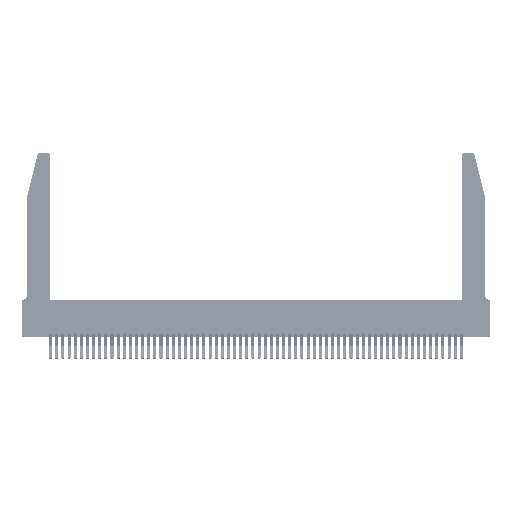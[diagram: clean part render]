
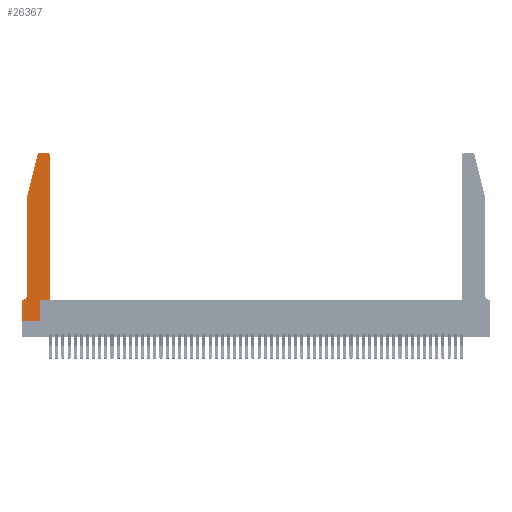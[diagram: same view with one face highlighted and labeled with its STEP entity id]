
A CAD part, top view. The second image highlights one B-rep face of the part: STEP entity #26367.
In plain terms, the highlighted planar face has unit normal (0, 0, 1).
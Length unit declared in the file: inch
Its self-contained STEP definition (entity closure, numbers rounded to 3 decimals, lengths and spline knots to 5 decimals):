
#1747 = ORIENTED_EDGE ( 'NONE', *, *, #37075, .T. ) ;
#2372 = VECTOR ( 'NONE', #35628, 39.37008 ) ;
#2471 = CARTESIAN_POINT ( 'NONE',  ( 0., 0.35, 0.37 ) ) ;
#2903 = CARTESIAN_POINT ( 'NONE',  ( 0.284, 2.72, 0.37 ) ) ;
#3510 = LINE ( 'NONE', #19784, #26291 ) ;
#3639 = DIRECTION ( 'NONE',  ( 0., -1., 0. ) ) ;
#5743 = VERTEX_POINT ( 'NONE', #14282 ) ;
#6787 = DIRECTION ( 'NONE',  ( 1., 0., 0. ) ) ;
#7068 = CARTESIAN_POINT ( 'NONE',  ( 0., 0., 0.37 ) ) ;
#7087 = CIRCLE ( 'NONE', #29695, 0.03 ) ;
#7235 = DIRECTION ( 'NONE',  ( 1., 0., 0. ) ) ;
#7266 = ORIENTED_EDGE ( 'NONE', *, *, #21138, .T. ) ;
#8142 = VECTOR ( 'NONE', #20509, 39.37008 ) ;
#8736 = CIRCLE ( 'NONE', #43316, 0.03 ) ;
#9038 = CARTESIAN_POINT ( 'NONE',  ( 0.4205, 2.72, 0.37 ) ) ;
#10412 = LINE ( 'NONE', #54182, #31751 ) ;
#11208 = VERTEX_POINT ( 'NONE', #11891 ) ;
#11594 = LINE ( 'NONE', #49987, #32873 ) ;
#11891 = CARTESIAN_POINT ( 'NONE',  ( 0., 0.35, 0.37 ) ) ;
#13338 = VERTEX_POINT ( 'NONE', #21195 ) ;
#13393 = DIRECTION ( 'NONE',  ( 1., 0., 0. ) ) ;
#13428 = DIRECTION ( 'NONE',  ( 0., 1., 0. ) ) ;
#13466 = ORIENTED_EDGE ( 'NONE', *, *, #21607, .T. ) ;
#14282 = CARTESIAN_POINT ( 'NONE',  ( 0.0055, 0.35, 0.37 ) ) ;
#15127 = CARTESIAN_POINT ( 'NONE',  ( 0.4205, 2.75, 0.37 ) ) ;
#15251 = CARTESIAN_POINT ( 'NONE',  ( 0.4505, 2.72, 0.37 ) ) ;
#15468 = VERTEX_POINT ( 'NONE', #19842 ) ;
#15907 = CIRCLE ( 'NONE', #34922, 0.07 ) ;
#16076 = ORIENTED_EDGE ( 'NONE', *, *, #27579, .T. ) ;
#16185 = CARTESIAN_POINT ( 'NONE',  ( 0.4505, 0.35, 0.37 ) ) ;
#16441 = LINE ( 'NONE', #17793, #37556 ) ;
#16730 = ORIENTED_EDGE ( 'NONE', *, *, #29113, .T. ) ;
#17793 = CARTESIAN_POINT ( 'NONE',  ( 0.2865, 0.35, 0.37 ) ) ;
#18177 = VERTEX_POINT ( 'NONE', #22594 ) ;
#18274 = DIRECTION ( 'NONE',  ( 0., 0., -1. ) ) ;
#19784 = CARTESIAN_POINT ( 'NONE',  ( 0.4505, 0.35, 0.37 ) ) ;
#19842 = CARTESIAN_POINT ( 'NONE',  ( 0.0755, 2., 0.37 ) ) ;
#19900 = VECTOR ( 'NONE', #41051, 39.37008 ) ;
#20276 = DIRECTION ( 'NONE',  ( 1., 0., 0. ) ) ;
#20509 = DIRECTION ( 'NONE',  ( 1., 0., 0. ) ) ;
#21038 = EDGE_CURVE ( 'NONE', #5743, #11208, #21962, .T. ) ;
#21138 = EDGE_CURVE ( 'NONE', #36410, #13338, #39012, .T. ) ;
#21195 = CARTESIAN_POINT ( 'NONE',  ( 0.2865, 0., 0.37 ) ) ;
#21607 = EDGE_CURVE ( 'NONE', #21693, #39519, #36318, .T. ) ;
#21693 = VERTEX_POINT ( 'NONE', #15127 ) ;
#21962 = LINE ( 'NONE', #28022, #45532 ) ;
#22594 = CARTESIAN_POINT ( 'NONE',  ( 0.25487, 2.72718, 0.37 ) ) ;
#23881 = PLANE ( 'NONE',  #51982 ) ;
#26291 = VECTOR ( 'NONE', #49035, 39.37008 ) ;
#26367 = ADVANCED_FACE ( 'NONE', ( #46452 ), #23881, .T. ) ;
#27579 = EDGE_CURVE ( 'NONE', #37062, #21693, #8736, .T. ) ;
#27873 = VECTOR ( 'NONE', #20276, 39.37008 ) ;
#28022 = CARTESIAN_POINT ( 'NONE',  ( 0.0755, 0.35, 0.37 ) ) ;
#29113 = EDGE_CURVE ( 'NONE', #39519, #18177, #7087, .T. ) ;
#29274 = EDGE_CURVE ( 'NONE', #11208, #36410, #10412, .T. ) ;
#29695 = AXIS2_PLACEMENT_3D ( 'NONE', #2903, #32740, #7235 ) ;
#29817 = VERTEX_POINT ( 'NONE', #43729 ) ;
#31404 = EDGE_CURVE ( 'NONE', #45785, #36505, #54282, .T. ) ;
#31453 = CARTESIAN_POINT ( 'NONE',  ( 0.2605, 2.75, 0.37 ) ) ;
#31751 = VECTOR ( 'NONE', #3639, 39.37008 ) ;
#32250 = DIRECTION ( 'NONE',  ( -1., 0., 0. ) ) ;
#32334 = DIRECTION ( 'NONE',  ( 0., 0., 1. ) ) ;
#32740 = DIRECTION ( 'NONE',  ( 0., 0., 1. ) ) ;
#32873 = VECTOR ( 'NONE', #54160, 39.37008 ) ;
#32877 = ORIENTED_EDGE ( 'NONE', *, *, #36154, .T. ) ;
#34922 = AXIS2_PLACEMENT_3D ( 'NONE', #43428, #18274, #47604 ) ;
#35380 = ORIENTED_EDGE ( 'NONE', *, *, #31404, .T. ) ;
#35379 = ORIENTED_EDGE ( 'NONE', *, *, #29274, .T. ) ;
#35628 = DIRECTION ( 'NONE',  ( -1., 0., 0. ) ) ;
#36154 = EDGE_CURVE ( 'NONE', #13338, #45785, #16441, .T. ) ;
#36318 = LINE ( 'NONE', #31453, #2372 ) ;
#36410 = VERTEX_POINT ( 'NONE', #44742 ) ;
#36505 = VERTEX_POINT ( 'NONE', #49458 ) ;
#37062 = VERTEX_POINT ( 'NONE', #15251 ) ;
#37075 = EDGE_CURVE ( 'NONE', #36505, #37062, #3510, .T. ) ;
#37556 = VECTOR ( 'NONE', #13428, 39.37008 ) ;
#38142 = ORIENTED_EDGE ( 'NONE', *, *, #53994, .T. ) ;
#38730 = DIRECTION ( 'NONE',  ( 0., 0., 1. ) ) ;
#39012 = LINE ( 'NONE', #7068, #27873 ) ;
#39519 = VERTEX_POINT ( 'NONE', #39595 ) ;
#39595 = CARTESIAN_POINT ( 'NONE',  ( 0.284, 2.75, 0.37 ) ) ;
#41051 = DIRECTION ( 'NONE',  ( -0.239, -0.971, 0. ) ) ;
#42082 = EDGE_LOOP ( 'NONE', ( #13466, #16730, #44200, #42356, #38142, #49148, #35379, #7266, #32877, #35380, #1747, #16076 ) ) ;
#42356 = ORIENTED_EDGE ( 'NONE', *, *, #42972, .T. ) ;
#42972 = EDGE_CURVE ( 'NONE', #15468, #29817, #11594, .T. ) ;
#43316 = AXIS2_PLACEMENT_3D ( 'NONE', #9038, #38730, #13393 ) ;
#43428 = CARTESIAN_POINT ( 'NONE',  ( 0.0055, 0.42, 0.37 ) ) ;
#43729 = CARTESIAN_POINT ( 'NONE',  ( 0.0755, 0.42, 0.37 ) ) ;
#44200 = ORIENTED_EDGE ( 'NONE', *, *, #54297, .T. ) ;
#44742 = CARTESIAN_POINT ( 'NONE',  ( 0., 0., 0.37 ) ) ;
#44947 = CARTESIAN_POINT ( 'NONE',  ( 0.2865, 0.35, 0.37 ) ) ;
#45038 = CARTESIAN_POINT ( 'NONE',  ( 0.0755, 2., 0.37 ) ) ;
#45532 = VECTOR ( 'NONE', #32250, 39.37008 ) ;
#45785 = VERTEX_POINT ( 'NONE', #44947 ) ;
#46452 = FACE_OUTER_BOUND ( 'NONE', #42082, .T. ) ;
#47604 = DIRECTION ( 'NONE',  ( -1., 0., 0. ) ) ;
#49035 = DIRECTION ( 'NONE',  ( 0., 1., 0. ) ) ;
#49148 = ORIENTED_EDGE ( 'NONE', *, *, #21038, .T. ) ;
#49458 = CARTESIAN_POINT ( 'NONE',  ( 0.4505, 0.35, 0.37 ) ) ;
#49987 = CARTESIAN_POINT ( 'NONE',  ( 0.0755, 2., 0.37 ) ) ;
#51982 = AXIS2_PLACEMENT_3D ( 'NONE', #2471, #32334, #6787 ) ;
#53242 = LINE ( 'NONE', #45038, #19900 ) ;
#53994 = EDGE_CURVE ( 'NONE', #29817, #5743, #15907, .T. ) ;
#54160 = DIRECTION ( 'NONE',  ( 0., -1., 0. ) ) ;
#54182 = CARTESIAN_POINT ( 'NONE',  ( 0., 0., 0.37 ) ) ;
#54282 = LINE ( 'NONE', #16185, #8142 ) ;
#54297 = EDGE_CURVE ( 'NONE', #18177, #15468, #53242, .T. ) ;
